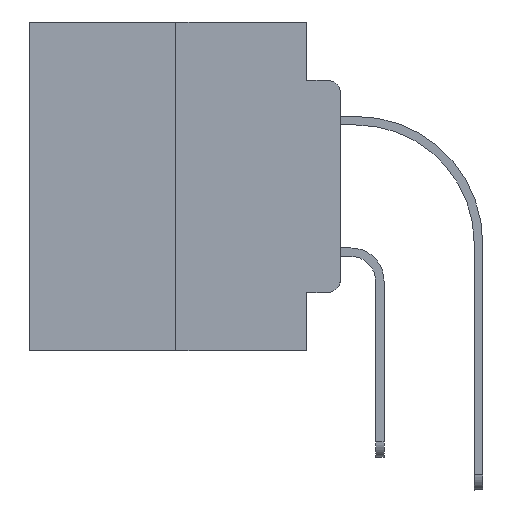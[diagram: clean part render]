
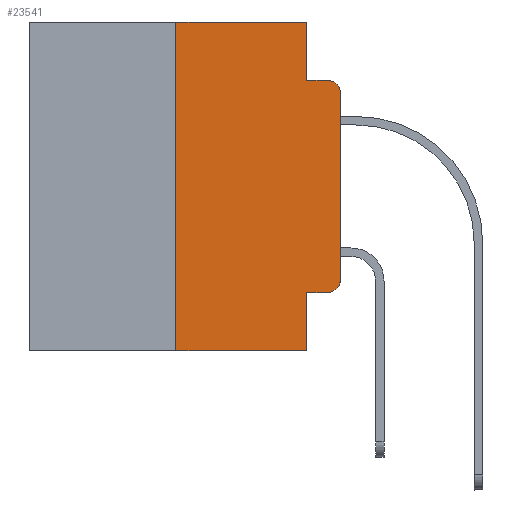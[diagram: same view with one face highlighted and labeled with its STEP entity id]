
A CAD part, left-side view. The second image highlights one B-rep face of the part: STEP entity #23541.
In plain terms, the highlighted planar face has unit normal (-1, 0, 0).
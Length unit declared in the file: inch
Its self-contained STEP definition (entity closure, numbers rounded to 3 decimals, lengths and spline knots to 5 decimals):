
#4 = VERTEX_POINT ( 'NONE', #1901 ) ;
#684 = ORIENTED_EDGE ( 'NONE', *, *, #12701, .F. ) ;
#1135 = CARTESIAN_POINT ( 'NONE',  ( 0., 0.25, -0.5 ) ) ;
#1184 = VECTOR ( 'NONE', #27775, 39.37008 ) ;
#1901 = CARTESIAN_POINT ( 'NONE',  ( 0., 0., -0.3915 ) ) ;
#1999 = EDGE_CURVE ( 'NONE', #8983, #19242, #16401, .T. ) ;
#2103 = CARTESIAN_POINT ( 'NONE',  ( 0., 0.051, 0. ) ) ;
#2507 = VECTOR ( 'NONE', #9620, 39.37008 ) ;
#3168 = LINE ( 'NONE', #10155, #1184 ) ;
#3308 = VERTEX_POINT ( 'NONE', #12413 ) ;
#3719 = CARTESIAN_POINT ( 'NONE',  ( 0., 0.473, 0. ) ) ;
#3890 = DIRECTION ( 'NONE',  ( 0., 0., -1. ) ) ;
#3900 = VERTEX_POINT ( 'NONE', #28064 ) ;
#4722 = CARTESIAN_POINT ( 'NONE',  ( 0., 0.02, -0.1085 ) ) ;
#5256 = EDGE_CURVE ( 'NONE', #22615, #17447, #3168, .T. ) ;
#5340 = EDGE_CURVE ( 'NONE', #22615, #3308, #15482, .T. ) ;
#5764 = AXIS2_PLACEMENT_3D ( 'NONE', #3719, #10710, #6097 ) ;
#6097 = DIRECTION ( 'NONE',  ( 0., 0., -1. ) ) ;
#6155 = CARTESIAN_POINT ( 'NONE',  ( 0., 0.051, -0.0885 ) ) ;
#6331 = ORIENTED_EDGE ( 'NONE', *, *, #22412, .F. ) ;
#6536 = CIRCLE ( 'NONE', #11289, 0.02 ) ;
#7068 = DIRECTION ( 'NONE',  ( 0., -1., 0. ) ) ;
#7723 = CIRCLE ( 'NONE', #15309, 0.02 ) ;
#8256 = LINE ( 'NONE', #16865, #27365 ) ;
#8330 = FACE_OUTER_BOUND ( 'NONE', #19715, .T. ) ;
#8363 = CARTESIAN_POINT ( 'NONE',  ( 0., 0.25, 0. ) ) ;
#8983 = VERTEX_POINT ( 'NONE', #6155 ) ;
#9620 = DIRECTION ( 'NONE',  ( 0., -1., 0. ) ) ;
#9734 = CARTESIAN_POINT ( 'NONE',  ( 0., 0.051, -0.4115 ) ) ;
#9866 = CARTESIAN_POINT ( 'NONE',  ( 0., 0., 0. ) ) ;
#10155 = CARTESIAN_POINT ( 'NONE',  ( 0., 0.473, -0.5 ) ) ;
#10494 = ORIENTED_EDGE ( 'NONE', *, *, #1999, .F. ) ;
#10710 = DIRECTION ( 'NONE',  ( 1., 0., 0. ) ) ;
#11289 = AXIS2_PLACEMENT_3D ( 'NONE', #4722, #22796, #21025 ) ;
#11481 = ORIENTED_EDGE ( 'NONE', *, *, #12544, .T. ) ;
#12413 = CARTESIAN_POINT ( 'NONE',  ( 0., 0.25, 0. ) ) ;
#12544 = EDGE_CURVE ( 'NONE', #17212, #19242, #6536, .T. ) ;
#12701 = EDGE_CURVE ( 'NONE', #24394, #8983, #8256, .T. ) ;
#12731 = DIRECTION ( 'NONE',  ( 0., 0., -1. ) ) ;
#12832 = VERTEX_POINT ( 'NONE', #28990 ) ;
#13235 = CARTESIAN_POINT ( 'NONE',  ( 0., 0., -0.1085 ) ) ;
#13379 = ORIENTED_EDGE ( 'NONE', *, *, #5340, .F. ) ;
#15172 = CARTESIAN_POINT ( 'NONE',  ( 0., 0.02, -0.3915 ) ) ;
#15309 = AXIS2_PLACEMENT_3D ( 'NONE', #15172, #24191, #3890 ) ;
#15374 = CARTESIAN_POINT ( 'NONE',  ( 0., 0.02, -0.0885 ) ) ;
#15482 = LINE ( 'NONE', #8363, #28650 ) ;
#15694 = ORIENTED_EDGE ( 'NONE', *, *, #21657, .T. ) ;
#16401 = LINE ( 'NONE', #16549, #23511 ) ;
#16549 = CARTESIAN_POINT ( 'NONE',  ( 0., 0.051, -0.0885 ) ) ;
#16635 = EDGE_CURVE ( 'NONE', #3900, #4, #7723, .T. ) ;
#16865 = CARTESIAN_POINT ( 'NONE',  ( 0., 0.051, 0. ) ) ;
#16934 = ORIENTED_EDGE ( 'NONE', *, *, #16635, .T. ) ;
#17212 = VERTEX_POINT ( 'NONE', #13235 ) ;
#17447 = VERTEX_POINT ( 'NONE', #28421 ) ;
#18498 = LINE ( 'NONE', #25454, #2507 ) ;
#19242 = VERTEX_POINT ( 'NONE', #15374 ) ;
#19715 = EDGE_LOOP ( 'NONE', ( #15694, #11481, #10494, #684, #6331, #13379, #23099, #24804, #27515, #16934 ) ) ;
#21025 = DIRECTION ( 'NONE',  ( 0., 0., -1. ) ) ;
#21657 = EDGE_CURVE ( 'NONE', #4, #17212, #28065, .T. ) ;
#22412 = EDGE_CURVE ( 'NONE', #3308, #24394, #18498, .T. ) ;
#22615 = VERTEX_POINT ( 'NONE', #1135 ) ;
#22796 = DIRECTION ( 'NONE',  ( -1., 0., 0. ) ) ;
#23099 = ORIENTED_EDGE ( 'NONE', *, *, #5256, .T. ) ;
#23511 = VECTOR ( 'NONE', #25429, 39.37008 ) ;
#23541 = ADVANCED_FACE ( 'NONE', ( #8330 ), #24625, .F. ) ;
#23621 = DIRECTION ( 'NONE',  ( 0., 0., 1. ) ) ;
#23885 = VECTOR ( 'NONE', #26406, 39.37008 ) ;
#24068 = CARTESIAN_POINT ( 'NONE',  ( 0., 0.051, 0. ) ) ;
#24191 = DIRECTION ( 'NONE',  ( -1., 0., 0. ) ) ;
#24394 = VERTEX_POINT ( 'NONE', #24068 ) ;
#24532 = VECTOR ( 'NONE', #7068, 39.37008 ) ;
#24625 = PLANE ( 'NONE',  #5764 ) ;
#24659 = EDGE_CURVE ( 'NONE', #12832, #17447, #27005, .T. ) ;
#24804 = ORIENTED_EDGE ( 'NONE', *, *, #24659, .F. ) ;
#25429 = DIRECTION ( 'NONE',  ( 0., -1., 0. ) ) ;
#25433 = LINE ( 'NONE', #9734, #24532 ) ;
#25454 = CARTESIAN_POINT ( 'NONE',  ( 0., 0.473, 0. ) ) ;
#26406 = DIRECTION ( 'NONE',  ( 0., 0., -1. ) ) ;
#27005 = LINE ( 'NONE', #2103, #23885 ) ;
#27109 = VECTOR ( 'NONE', #23621, 39.37008 ) ;
#27365 = VECTOR ( 'NONE', #12731, 39.37008 ) ;
#27515 = ORIENTED_EDGE ( 'NONE', *, *, #28966, .T. ) ;
#27775 = DIRECTION ( 'NONE',  ( 0., -1., 0. ) ) ;
#28064 = CARTESIAN_POINT ( 'NONE',  ( 0., 0.02, -0.4115 ) ) ;
#28065 = LINE ( 'NONE', #9866, #27109 ) ;
#28421 = CARTESIAN_POINT ( 'NONE',  ( 0., 0.051, -0.5 ) ) ;
#28645 = DIRECTION ( 'NONE',  ( 0., 0., 1. ) ) ;
#28650 = VECTOR ( 'NONE', #28645, 39.37008 ) ;
#28966 = EDGE_CURVE ( 'NONE', #12832, #3900, #25433, .T. ) ;
#28990 = CARTESIAN_POINT ( 'NONE',  ( 0., 0.051, -0.4115 ) ) ;
